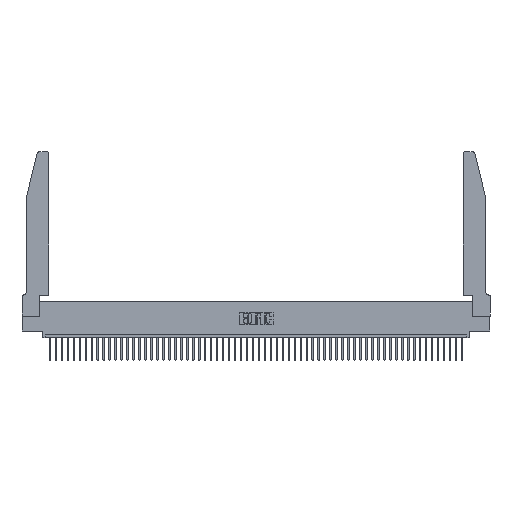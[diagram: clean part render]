
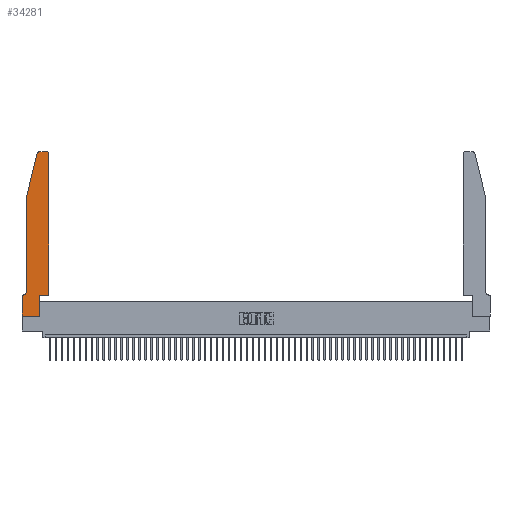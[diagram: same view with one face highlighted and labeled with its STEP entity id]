
A CAD part, top view. The second image highlights one B-rep face of the part: STEP entity #34281.
In plain terms, the highlighted planar face has unit normal (0, 0, 1).
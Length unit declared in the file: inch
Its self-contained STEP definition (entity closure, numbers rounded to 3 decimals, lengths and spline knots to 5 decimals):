
#521 = EDGE_CURVE ( 'NONE', #36935, #15758, #39111, .T. ) ;
#567 = EDGE_CURVE ( 'NONE', #19335, #28824, #50712, .T. ) ;
#1190 = ORIENTED_EDGE ( 'NONE', *, *, #521, .T. ) ;
#1973 = CARTESIAN_POINT ( 'NONE',  ( 0.0755, 0.42, 0.37 ) ) ;
#2610 = EDGE_CURVE ( 'NONE', #14529, #16519, #42678, .T. ) ;
#3058 = DIRECTION ( 'NONE',  ( 0., 0., 1. ) ) ;
#3733 = VECTOR ( 'NONE', #16884, 39.37008 ) ;
#4929 = EDGE_CURVE ( 'NONE', #33991, #19335, #11326, .T. ) ;
#5399 = ORIENTED_EDGE ( 'NONE', *, *, #4929, .T. ) ;
#5534 = VERTEX_POINT ( 'NONE', #17926 ) ;
#5575 = VECTOR ( 'NONE', #35060, 39.37008 ) ;
#5935 = DIRECTION ( 'NONE',  ( 0., 0., 1. ) ) ;
#6419 = DIRECTION ( 'NONE',  ( 0., 0., 1. ) ) ;
#6675 = CARTESIAN_POINT ( 'NONE',  ( 0.284, 2.72, 0.37 ) ) ;
#6833 = ORIENTED_EDGE ( 'NONE', *, *, #37003, .T. ) ;
#7089 = FACE_OUTER_BOUND ( 'NONE', #13621, .T. ) ;
#7558 = DIRECTION ( 'NONE',  ( 0., -1., 0. ) ) ;
#7851 = VERTEX_POINT ( 'NONE', #19751 ) ;
#8188 = ORIENTED_EDGE ( 'NONE', *, *, #18824, .T. ) ;
#9622 = CIRCLE ( 'NONE', #18622, 0.03 ) ;
#9724 = EDGE_CURVE ( 'NONE', #5534, #10195, #38741, .T. ) ;
#9820 = EDGE_CURVE ( 'NONE', #28824, #7851, #13398, .T. ) ;
#10195 = VERTEX_POINT ( 'NONE', #23509 ) ;
#10703 = CARTESIAN_POINT ( 'NONE',  ( 0.2865, 0.35, 0.37 ) ) ;
#11033 = DIRECTION ( 'NONE',  ( 1., 0., 0. ) ) ;
#11134 = VECTOR ( 'NONE', #40378, 39.37008 ) ;
#11326 = LINE ( 'NONE', #47188, #12013 ) ;
#11895 = CARTESIAN_POINT ( 'NONE',  ( 0., 0., 0.37 ) ) ;
#12013 = VECTOR ( 'NONE', #17528, 39.37008 ) ;
#13097 = VERTEX_POINT ( 'NONE', #52076 ) ;
#13398 = LINE ( 'NONE', #33172, #3733 ) ;
#13621 = EDGE_LOOP ( 'NONE', ( #23078, #26996, #16062, #5399, #45780, #20109, #6833, #15643, #48697, #1190, #8188, #20496 ) ) ;
#13838 = EDGE_CURVE ( 'NONE', #13097, #33991, #18133, .T. ) ;
#14529 = VERTEX_POINT ( 'NONE', #32378 ) ;
#15643 = ORIENTED_EDGE ( 'NONE', *, *, #9724, .T. ) ;
#15751 = CARTESIAN_POINT ( 'NONE',  ( 0.4505, 0.35, 0.37 ) ) ;
#15758 = VERTEX_POINT ( 'NONE', #20043 ) ;
#16062 = ORIENTED_EDGE ( 'NONE', *, *, #13838, .T. ) ;
#16200 = VECTOR ( 'NONE', #7558, 39.37008 ) ;
#16519 = VERTEX_POINT ( 'NONE', #32039 ) ;
#16884 = DIRECTION ( 'NONE',  ( -1., 0., 0. ) ) ;
#17528 = DIRECTION ( 'NONE',  ( 0., -1., 0. ) ) ;
#17926 = CARTESIAN_POINT ( 'NONE',  ( 0., 0., 0.37 ) ) ;
#18133 = LINE ( 'NONE', #49725, #49978 ) ;
#18590 = PLANE ( 'NONE',  #19135 ) ;
#18622 = AXIS2_PLACEMENT_3D ( 'NONE', #6675, #3058, #11033 ) ;
#18824 = EDGE_CURVE ( 'NONE', #15758, #14529, #43588, .T. ) ;
#19135 = AXIS2_PLACEMENT_3D ( 'NONE', #22773, #6419, #22571 ) ;
#19335 = VERTEX_POINT ( 'NONE', #1973 ) ;
#19751 = CARTESIAN_POINT ( 'NONE',  ( 0., 0.35, 0.37 ) ) ;
#19990 = EDGE_CURVE ( 'NONE', #42911, #13097, #9622, .T. ) ;
#20043 = CARTESIAN_POINT ( 'NONE',  ( 0.4505, 0.35, 0.37 ) ) ;
#20109 = ORIENTED_EDGE ( 'NONE', *, *, #9820, .T. ) ;
#20496 = ORIENTED_EDGE ( 'NONE', *, *, #2610, .T. ) ;
#22571 = DIRECTION ( 'NONE',  ( 1., 0., 0. ) ) ;
#22773 = CARTESIAN_POINT ( 'NONE',  ( 0., 0.35, 0.37 ) ) ;
#23078 = ORIENTED_EDGE ( 'NONE', *, *, #53787, .T. ) ;
#23080 = DIRECTION ( 'NONE',  ( 0., 1., 0. ) ) ;
#23509 = CARTESIAN_POINT ( 'NONE',  ( 0.2865, 0., 0.37 ) ) ;
#23744 = DIRECTION ( 'NONE',  ( 0., 0., -1. ) ) ;
#24008 = LINE ( 'NONE', #11895, #16200 ) ;
#24691 = LINE ( 'NONE', #35367, #47942 ) ;
#26996 = ORIENTED_EDGE ( 'NONE', *, *, #19990, .T. ) ;
#27118 = CARTESIAN_POINT ( 'NONE',  ( 0.2605, 2.75, 0.37 ) ) ;
#27232 = DIRECTION ( 'NONE',  ( -0.239, -0.971, 0. ) ) ;
#27518 = AXIS2_PLACEMENT_3D ( 'NONE', #32477, #23744, #48721 ) ;
#28138 = DIRECTION ( 'NONE',  ( 1., 0., 0. ) ) ;
#28371 = LINE ( 'NONE', #27118, #39910 ) ;
#28824 = VERTEX_POINT ( 'NONE', #35520 ) ;
#32039 = CARTESIAN_POINT ( 'NONE',  ( 0.4205, 2.75, 0.37 ) ) ;
#32378 = CARTESIAN_POINT ( 'NONE',  ( 0.4505, 2.72, 0.37 ) ) ;
#32477 = CARTESIAN_POINT ( 'NONE',  ( 0.0055, 0.42, 0.37 ) ) ;
#33172 = CARTESIAN_POINT ( 'NONE',  ( 0.0755, 0.35, 0.37 ) ) ;
#33991 = VERTEX_POINT ( 'NONE', #34425 ) ;
#34281 = ADVANCED_FACE ( 'NONE', ( #7089 ), #18590, .T. ) ;
#34425 = CARTESIAN_POINT ( 'NONE',  ( 0.0755, 2., 0.37 ) ) ;
#35060 = DIRECTION ( 'NONE',  ( 1., 0., 0. ) ) ;
#35367 = CARTESIAN_POINT ( 'NONE',  ( 0.2865, 0.35, 0.37 ) ) ;
#35520 = CARTESIAN_POINT ( 'NONE',  ( 0.0055, 0.35, 0.37 ) ) ;
#36935 = VERTEX_POINT ( 'NONE', #10703 ) ;
#37003 = EDGE_CURVE ( 'NONE', #7851, #5534, #24008, .T. ) ;
#38741 = LINE ( 'NONE', #52140, #5575 ) ;
#39111 = LINE ( 'NONE', #15751, #44380 ) ;
#39910 = VECTOR ( 'NONE', #51706, 39.37008 ) ;
#40378 = DIRECTION ( 'NONE',  ( 0., 1., 0. ) ) ;
#40738 = EDGE_CURVE ( 'NONE', #10195, #36935, #24691, .T. ) ;
#42678 = CIRCLE ( 'NONE', #50094, 0.03 ) ;
#42911 = VERTEX_POINT ( 'NONE', #49668 ) ;
#43513 = CARTESIAN_POINT ( 'NONE',  ( 0.4205, 2.72, 0.37 ) ) ;
#43588 = LINE ( 'NONE', #52317, #11134 ) ;
#43905 = DIRECTION ( 'NONE',  ( 1., 0., 0. ) ) ;
#44380 = VECTOR ( 'NONE', #28138, 39.37008 ) ;
#45780 = ORIENTED_EDGE ( 'NONE', *, *, #567, .T. ) ;
#47188 = CARTESIAN_POINT ( 'NONE',  ( 0.0755, 2., 0.37 ) ) ;
#47942 = VECTOR ( 'NONE', #23080, 39.37008 ) ;
#48697 = ORIENTED_EDGE ( 'NONE', *, *, #40738, .T. ) ;
#48721 = DIRECTION ( 'NONE',  ( -1., 0., 0. ) ) ;
#49668 = CARTESIAN_POINT ( 'NONE',  ( 0.284, 2.75, 0.37 ) ) ;
#49725 = CARTESIAN_POINT ( 'NONE',  ( 0.0755, 2., 0.37 ) ) ;
#49978 = VECTOR ( 'NONE', #27232, 39.37008 ) ;
#50094 = AXIS2_PLACEMENT_3D ( 'NONE', #43513, #5935, #43905 ) ;
#50712 = CIRCLE ( 'NONE', #27518, 0.07 ) ;
#51706 = DIRECTION ( 'NONE',  ( -1., 0., 0. ) ) ;
#52076 = CARTESIAN_POINT ( 'NONE',  ( 0.25487, 2.72718, 0.37 ) ) ;
#52140 = CARTESIAN_POINT ( 'NONE',  ( 0., 0., 0.37 ) ) ;
#52317 = CARTESIAN_POINT ( 'NONE',  ( 0.4505, 0.35, 0.37 ) ) ;
#53787 = EDGE_CURVE ( 'NONE', #16519, #42911, #28371, .T. ) ;
